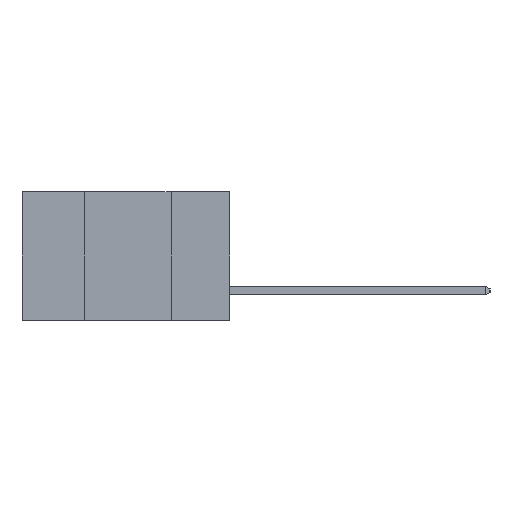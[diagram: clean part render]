
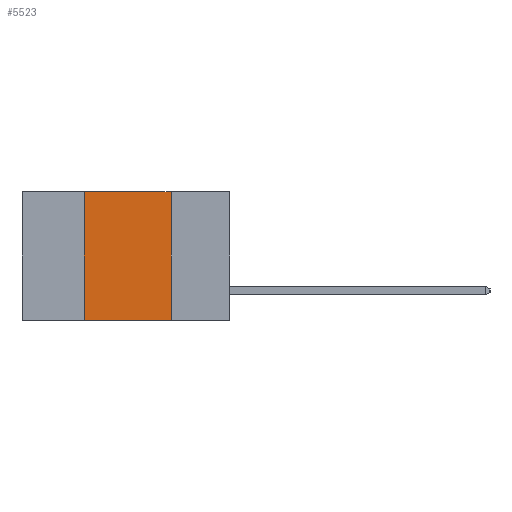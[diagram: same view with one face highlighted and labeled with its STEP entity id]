
A CAD part, left-side view. The second image highlights one B-rep face of the part: STEP entity #5523.
In plain terms, the highlighted planar face has unit normal (-1, 0, 0).
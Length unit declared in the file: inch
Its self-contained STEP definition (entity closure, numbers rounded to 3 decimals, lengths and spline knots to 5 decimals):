
#553 = DIRECTION ( 'NONE',  ( 0., 0., -1. ) ) ;
#569 = VERTEX_POINT ( 'NONE', #19213 ) ;
#1996 = CARTESIAN_POINT ( 'NONE',  ( 0., 0.6, 0. ) ) ;
#2805 = ORIENTED_EDGE ( 'NONE', *, *, #15573, .F. ) ;
#3130 = CARTESIAN_POINT ( 'NONE',  ( 0., 0.6, 0. ) ) ;
#4309 = VECTOR ( 'NONE', #11683, 39.37008 ) ;
#4720 = DIRECTION ( 'NONE',  ( 0., -1., 0. ) ) ;
#5407 = FACE_OUTER_BOUND ( 'NONE', #13251, .T. ) ;
#5523 = ADVANCED_FACE ( 'NONE', ( #5407 ), #19342, .F. ) ;
#6371 = DIRECTION ( 'NONE',  ( 0., 0., -1. ) ) ;
#6511 = EDGE_CURVE ( 'NONE', #10359, #9801, #8817, .T. ) ;
#7580 = EDGE_CURVE ( 'NONE', #10359, #569, #8504, .T. ) ;
#7726 = ORIENTED_EDGE ( 'NONE', *, *, #7580, .F. ) ;
#8504 = LINE ( 'NONE', #10146, #4309 ) ;
#8632 = EDGE_CURVE ( 'NONE', #13269, #9801, #16921, .T. ) ;
#8817 = LINE ( 'NONE', #10980, #12521 ) ;
#8999 = VECTOR ( 'NONE', #6371, 39.37008 ) ;
#9236 = CARTESIAN_POINT ( 'NONE',  ( 0., 0.17, 0. ) ) ;
#9801 = VERTEX_POINT ( 'NONE', #15049 ) ;
#9982 = DIRECTION ( 'NONE',  ( 1., 0., 0. ) ) ;
#10146 = CARTESIAN_POINT ( 'NONE',  ( 0., 0.42, 0. ) ) ;
#10345 = CARTESIAN_POINT ( 'NONE',  ( 0., 0.42, -0.37 ) ) ;
#10359 = VERTEX_POINT ( 'NONE', #10345 ) ;
#10980 = CARTESIAN_POINT ( 'NONE',  ( 0., 0.6, -0.37 ) ) ;
#11683 = DIRECTION ( 'NONE',  ( 0., 0., 1. ) ) ;
#12371 = VECTOR ( 'NONE', #4720, 39.37008 ) ;
#12521 = VECTOR ( 'NONE', #18780, 39.37008 ) ;
#13251 = EDGE_LOOP ( 'NONE', ( #17818, #2805, #7726, #15668 ) ) ;
#13269 = VERTEX_POINT ( 'NONE', #9236 ) ;
#15049 = CARTESIAN_POINT ( 'NONE',  ( 0., 0.17, -0.37 ) ) ;
#15573 = EDGE_CURVE ( 'NONE', #569, #13269, #16591, .T. ) ;
#15668 = ORIENTED_EDGE ( 'NONE', *, *, #6511, .T. ) ;
#15883 = CARTESIAN_POINT ( 'NONE',  ( 0., 0.17, 0. ) ) ;
#16591 = LINE ( 'NONE', #3130, #12371 ) ;
#16921 = LINE ( 'NONE', #15883, #8999 ) ;
#17818 = ORIENTED_EDGE ( 'NONE', *, *, #8632, .F. ) ;
#18745 = AXIS2_PLACEMENT_3D ( 'NONE', #1996, #9982, #553 ) ;
#18780 = DIRECTION ( 'NONE',  ( 0., -1., 0. ) ) ;
#19213 = CARTESIAN_POINT ( 'NONE',  ( 0., 0.42, 0. ) ) ;
#19342 = PLANE ( 'NONE',  #18745 ) ;
